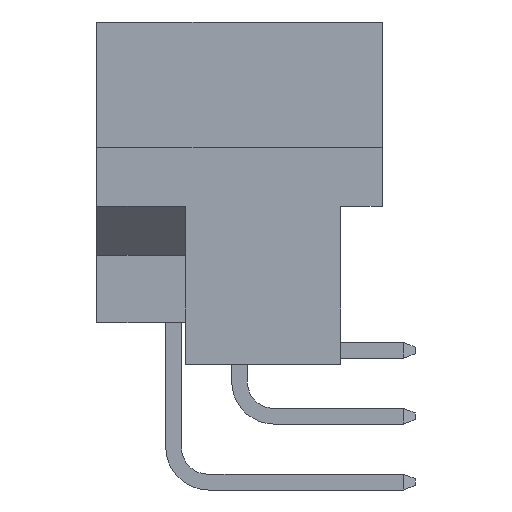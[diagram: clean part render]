
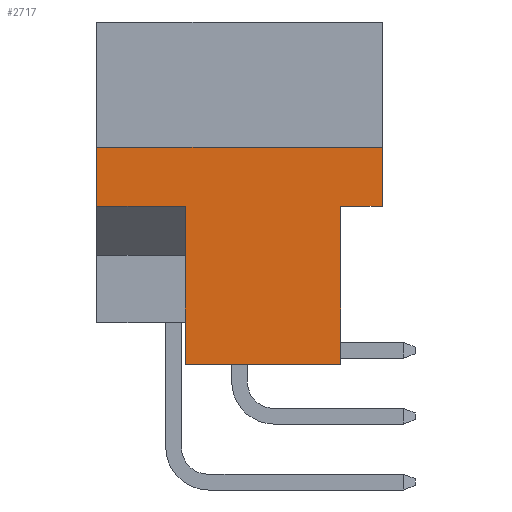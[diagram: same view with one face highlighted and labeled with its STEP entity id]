
A CAD part, left-side view. The second image highlights one B-rep face of the part: STEP entity #2717.
In plain terms, the highlighted planar face has unit normal (-1, 0, 0).
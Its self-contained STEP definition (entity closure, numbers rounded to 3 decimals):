
#292 = CARTESIAN_POINT ( 'NONE',  ( 0., 0., -4.826 ) ) ;
#391 = DIRECTION ( 'NONE',  ( 0., 0., 1. ) ) ;
#475 = VECTOR ( 'NONE', #6237, 1000. ) ;
#546 = EDGE_CURVE ( 'NONE', #3268, #7326, #4137, .T. ) ;
#613 = ORIENTED_EDGE ( 'NONE', *, *, #8011, .F. ) ;
#657 = CARTESIAN_POINT ( 'NONE',  ( 0., 10.998, 0. ) ) ;
#919 = ORIENTED_EDGE ( 'NONE', *, *, #5224, .T. ) ;
#925 = ORIENTED_EDGE ( 'NONE', *, *, #1001, .T. ) ;
#949 = VERTEX_POINT ( 'NONE', #292 ) ;
#1001 = EDGE_CURVE ( 'NONE', #8604, #949, #5648, .T. ) ;
#1595 = VECTOR ( 'NONE', #5515, 1000. ) ;
#1682 = VERTEX_POINT ( 'NONE', #8794 ) ;
#1686 = CARTESIAN_POINT ( 'NONE',  ( 0., 1.6, 46.912 ) ) ;
#1706 = CARTESIAN_POINT ( 'NONE',  ( 0., 7.597, -7.112 ) ) ;
#2372 = EDGE_CURVE ( 'NONE', #8671, #949, #8194, .T. ) ;
#2378 = LINE ( 'NONE', #4622, #6681 ) ;
#2411 = ORIENTED_EDGE ( 'NONE', *, *, #2372, .F. ) ;
#2572 = DIRECTION ( 'NONE',  ( 0., 1., 0. ) ) ;
#2606 = DIRECTION ( 'NONE',  ( 0., -1., 0. ) ) ;
#2612 = CARTESIAN_POINT ( 'NONE',  ( 0., 0., -7.112 ) ) ;
#2707 = CARTESIAN_POINT ( 'NONE',  ( 0., 10.998, -4.826 ) ) ;
#2717 = ADVANCED_FACE ( 'NONE', ( #8403 ), #7626, .F. ) ;
#2768 = VECTOR ( 'NONE', #391, 1000. ) ;
#2965 = CARTESIAN_POINT ( 'NONE',  ( 0., 7.597, -7.112 ) ) ;
#3166 = AXIS2_PLACEMENT_3D ( 'NONE', #9988, #8355, #6797 ) ;
#3167 = ORIENTED_EDGE ( 'NONE', *, *, #9790, .F. ) ;
#3268 = VERTEX_POINT ( 'NONE', #7766 ) ;
#3422 = VERTEX_POINT ( 'NONE', #8747 ) ;
#3735 = VERTEX_POINT ( 'NONE', #2965 ) ;
#4054 = VECTOR ( 'NONE', #9304, 1000. ) ;
#4104 = LINE ( 'NONE', #1706, #7332 ) ;
#4137 = LINE ( 'NONE', #1686, #1595 ) ;
#4560 = LINE ( 'NONE', #7684, #475 ) ;
#4622 = CARTESIAN_POINT ( 'NONE',  ( 0., 7.597, -13.2 ) ) ;
#4822 = CARTESIAN_POINT ( 'NONE',  ( 0., 10.998, -13.2 ) ) ;
#4930 = CARTESIAN_POINT ( 'NONE',  ( 0., 0., 0. ) ) ;
#5224 = EDGE_CURVE ( 'NONE', #3422, #7326, #5584, .T. ) ;
#5405 = EDGE_LOOP ( 'NONE', ( #6072, #8675, #925, #2411, #6596, #613, #3167, #919 ) ) ;
#5474 = VECTOR ( 'NONE', #5539, 1000. ) ;
#5515 = DIRECTION ( 'NONE',  ( 0., 0., -1. ) ) ;
#5539 = DIRECTION ( 'NONE',  ( 0., -1., 0. ) ) ;
#5584 = LINE ( 'NONE', #4822, #5474 ) ;
#5648 = LINE ( 'NONE', #4930, #2768 ) ;
#6072 = ORIENTED_EDGE ( 'NONE', *, *, #546, .F. ) ;
#6237 = DIRECTION ( 'NONE',  ( 0., 1., 0. ) ) ;
#6596 = ORIENTED_EDGE ( 'NONE', *, *, #7380, .F. ) ;
#6681 = VECTOR ( 'NONE', #9248, 1000. ) ;
#6797 = DIRECTION ( 'NONE',  ( 0., 0., -1. ) ) ;
#6983 = CARTESIAN_POINT ( 'NONE',  ( 0., 1.6, -13.2 ) ) ;
#7039 = EDGE_CURVE ( 'NONE', #8604, #3268, #4560, .T. ) ;
#7326 = VERTEX_POINT ( 'NONE', #6983 ) ;
#7332 = VECTOR ( 'NONE', #2572, 1000. ) ;
#7380 = EDGE_CURVE ( 'NONE', #1682, #8671, #7655, .T. ) ;
#7626 = PLANE ( 'NONE',  #3166 ) ;
#7655 = LINE ( 'NONE', #657, #4054 ) ;
#7684 = CARTESIAN_POINT ( 'NONE',  ( 0., 0., -7.112 ) ) ;
#7766 = CARTESIAN_POINT ( 'NONE',  ( 0., 1.6, -7.112 ) ) ;
#8011 = EDGE_CURVE ( 'NONE', #3735, #1682, #4104, .T. ) ;
#8194 = LINE ( 'NONE', #2707, #8711 ) ;
#8355 = DIRECTION ( 'NONE',  ( 1., 0., 0. ) ) ;
#8403 = FACE_OUTER_BOUND ( 'NONE', #5405, .T. ) ;
#8604 = VERTEX_POINT ( 'NONE', #2612 ) ;
#8671 = VERTEX_POINT ( 'NONE', #9111 ) ;
#8675 = ORIENTED_EDGE ( 'NONE', *, *, #7039, .F. ) ;
#8711 = VECTOR ( 'NONE', #2606, 1000. ) ;
#8747 = CARTESIAN_POINT ( 'NONE',  ( 0., 7.597, -13.2 ) ) ;
#8794 = CARTESIAN_POINT ( 'NONE',  ( 0., 10.998, -7.112 ) ) ;
#9111 = CARTESIAN_POINT ( 'NONE',  ( 0., 10.998, -4.826 ) ) ;
#9248 = DIRECTION ( 'NONE',  ( 0., 0., 1. ) ) ;
#9304 = DIRECTION ( 'NONE',  ( 0., 0., 1. ) ) ;
#9790 = EDGE_CURVE ( 'NONE', #3422, #3735, #2378, .T. ) ;
#9988 = CARTESIAN_POINT ( 'NONE',  ( 0., 10.998, 0. ) ) ;
